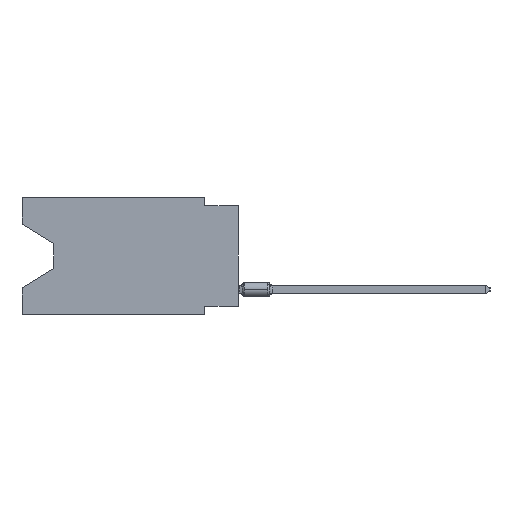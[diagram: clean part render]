
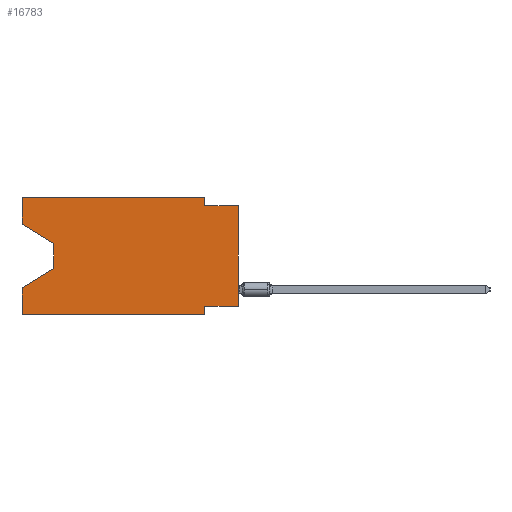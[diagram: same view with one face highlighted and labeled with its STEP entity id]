
A CAD part, left-side view. The second image highlights one B-rep face of the part: STEP entity #16783.
In plain terms, the highlighted planar face has unit normal (-1, 0, 0).
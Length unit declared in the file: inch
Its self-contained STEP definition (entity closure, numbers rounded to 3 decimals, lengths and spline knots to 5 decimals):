
#1095 = CARTESIAN_POINT ( 'NONE',  ( 0., 0.645, -0.08025 ) ) ;
#1118 = DIRECTION ( 'NONE',  ( 1., 0., 0. ) ) ;
#2425 = LINE ( 'NONE', #16137, #8555 ) ;
#2552 = ORIENTED_EDGE ( 'NONE', *, *, #15992, .T. ) ;
#2646 = ORIENTED_EDGE ( 'NONE', *, *, #29929, .T. ) ;
#3813 = VERTEX_POINT ( 'NONE', #6729 ) ;
#3839 = EDGE_CURVE ( 'NONE', #11808, #28434, #25571, .T. ) ;
#3952 = ORIENTED_EDGE ( 'NONE', *, *, #35474, .F. ) ;
#4165 = LINE ( 'NONE', #7543, #12275 ) ;
#4410 = VECTOR ( 'NONE', #7138, 39.37008 ) ;
#4477 = VERTEX_POINT ( 'NONE', #25203 ) ;
#5795 = VERTEX_POINT ( 'NONE', #40261 ) ;
#6729 = CARTESIAN_POINT ( 'NONE',  ( 0., 0.645, -0.35 ) ) ;
#7031 = CARTESIAN_POINT ( 'NONE',  ( 0., 0.1, -0.325 ) ) ;
#7138 = DIRECTION ( 'NONE',  ( 0., 0.855, -0.519 ) ) ;
#7151 = VECTOR ( 'NONE', #32783, 39.37008 ) ;
#7543 = CARTESIAN_POINT ( 'NONE',  ( 0., 0., -0.325 ) ) ;
#7919 = VECTOR ( 'NONE', #15474, 39.37008 ) ;
#8436 = VERTEX_POINT ( 'NONE', #17991 ) ;
#8555 = VECTOR ( 'NONE', #9391, 39.37008 ) ;
#8672 = DIRECTION ( 'NONE',  ( 0., 0., -1. ) ) ;
#9215 = LINE ( 'NONE', #25843, #41463 ) ;
#9391 = DIRECTION ( 'NONE',  ( 0., -1., 0. ) ) ;
#9828 = CARTESIAN_POINT ( 'NONE',  ( 0., 0.645, -0.35 ) ) ;
#10134 = VECTOR ( 'NONE', #16498, 39.37008 ) ;
#10283 = EDGE_CURVE ( 'NONE', #28434, #26085, #20039, .T. ) ;
#11442 = DIRECTION ( 'NONE',  ( 0., 0., -1. ) ) ;
#11808 = VERTEX_POINT ( 'NONE', #31929 ) ;
#11951 = LINE ( 'NONE', #22292, #36315 ) ;
#12116 = EDGE_CURVE ( 'NONE', #3813, #20471, #11951, .T. ) ;
#12165 = VERTEX_POINT ( 'NONE', #12174 ) ;
#12174 = CARTESIAN_POINT ( 'NONE',  ( 0., 0., -0.025 ) ) ;
#12275 = VECTOR ( 'NONE', #17874, 39.37008 ) ;
#12351 = LINE ( 'NONE', #16397, #17663 ) ;
#14331 = CARTESIAN_POINT ( 'NONE',  ( 0., 0.55, -0.212 ) ) ;
#14391 = EDGE_LOOP ( 'NONE', ( #43302, #19746, #2552, #34484, #2646, #43691, #32975, #43054, #3952, #27540, #29737, #34236 ) ) ;
#15425 = CARTESIAN_POINT ( 'NONE',  ( 0., 0.1, 0. ) ) ;
#15474 = DIRECTION ( 'NONE',  ( 0., -0.855, -0.519 ) ) ;
#15992 = EDGE_CURVE ( 'NONE', #26085, #20471, #37938, .T. ) ;
#16137 = CARTESIAN_POINT ( 'NONE',  ( 0., 0.645, 0. ) ) ;
#16397 = CARTESIAN_POINT ( 'NONE',  ( 0., 0., -0.025 ) ) ;
#16498 = DIRECTION ( 'NONE',  ( 0., 0., -1. ) ) ;
#16783 = ADVANCED_FACE ( 'NONE', ( #21348 ), #28104, .F. ) ;
#16889 = EDGE_CURVE ( 'NONE', #11808, #43099, #33010, .T. ) ;
#17663 = VECTOR ( 'NONE', #26286, 39.37008 ) ;
#17874 = DIRECTION ( 'NONE',  ( 0., 1., 0. ) ) ;
#17991 = CARTESIAN_POINT ( 'NONE',  ( 0., 0.1, -0.025 ) ) ;
#18970 = CARTESIAN_POINT ( 'NONE',  ( 0., 0.645, -0.26975 ) ) ;
#19081 = CARTESIAN_POINT ( 'NONE',  ( 0., 0.645, 0. ) ) ;
#19099 = DIRECTION ( 'NONE',  ( 0., 0., 1. ) ) ;
#19746 = ORIENTED_EDGE ( 'NONE', *, *, #10283, .T. ) ;
#20039 = LINE ( 'NONE', #20257, #42681 ) ;
#20257 = CARTESIAN_POINT ( 'NONE',  ( 0., 0.55, -0.138 ) ) ;
#20348 = EDGE_CURVE ( 'NONE', #4477, #39757, #4165, .T. ) ;
#20417 = EDGE_CURVE ( 'NONE', #39757, #23205, #22569, .T. ) ;
#20471 = VERTEX_POINT ( 'NONE', #18970 ) ;
#20620 = CARTESIAN_POINT ( 'NONE',  ( 0., 0.645, 0. ) ) ;
#20671 = VECTOR ( 'NONE', #8672, 39.37008 ) ;
#20800 = AXIS2_PLACEMENT_3D ( 'NONE', #31906, #1118, #11442 ) ;
#21058 = LINE ( 'NONE', #9828, #32996 ) ;
#21348 = FACE_OUTER_BOUND ( 'NONE', #14391, .T. ) ;
#21629 = DIRECTION ( 'NONE',  ( 0., 0., 1. ) ) ;
#22292 = CARTESIAN_POINT ( 'NONE',  ( 0., 0.645, 0. ) ) ;
#22569 = LINE ( 'NONE', #25938, #10134 ) ;
#23205 = VERTEX_POINT ( 'NONE', #41744 ) ;
#23768 = DIRECTION ( 'NONE',  ( 0., -1., 0. ) ) ;
#25203 = CARTESIAN_POINT ( 'NONE',  ( 0., 0., -0.325 ) ) ;
#25571 = LINE ( 'NONE', #1095, #7919 ) ;
#25843 = CARTESIAN_POINT ( 'NONE',  ( 0., 0., 0. ) ) ;
#25938 = CARTESIAN_POINT ( 'NONE',  ( 0., 0.1, -0.35 ) ) ;
#26085 = VERTEX_POINT ( 'NONE', #39390 ) ;
#26286 = DIRECTION ( 'NONE',  ( 0., -1., 0. ) ) ;
#26976 = CARTESIAN_POINT ( 'NONE',  ( 0., 0.55, -0.138 ) ) ;
#27540 = ORIENTED_EDGE ( 'NONE', *, *, #38713, .F. ) ;
#28104 = PLANE ( 'NONE',  #20800 ) ;
#28434 = VERTEX_POINT ( 'NONE', #26976 ) ;
#29579 = LINE ( 'NONE', #15425, #20671 ) ;
#29662 = EDGE_CURVE ( 'NONE', #43099, #5795, #2425, .T. ) ;
#29737 = ORIENTED_EDGE ( 'NONE', *, *, #29662, .F. ) ;
#29929 = EDGE_CURVE ( 'NONE', #3813, #23205, #21058, .T. ) ;
#31906 = CARTESIAN_POINT ( 'NONE',  ( 0., 0.645, 0. ) ) ;
#31929 = CARTESIAN_POINT ( 'NONE',  ( 0., 0.645, -0.08025 ) ) ;
#32783 = DIRECTION ( 'NONE',  ( 0., 0., 1. ) ) ;
#32975 = ORIENTED_EDGE ( 'NONE', *, *, #20348, .F. ) ;
#32996 = VECTOR ( 'NONE', #23768, 39.37008 ) ;
#33010 = LINE ( 'NONE', #19081, #7151 ) ;
#34236 = ORIENTED_EDGE ( 'NONE', *, *, #16889, .F. ) ;
#34484 = ORIENTED_EDGE ( 'NONE', *, *, #12116, .F. ) ;
#35474 = EDGE_CURVE ( 'NONE', #8436, #12165, #12351, .T. ) ;
#36315 = VECTOR ( 'NONE', #21629, 39.37008 ) ;
#36648 = EDGE_CURVE ( 'NONE', #4477, #12165, #9215, .T. ) ;
#36668 = DIRECTION ( 'NONE',  ( 0., 0., -1. ) ) ;
#37938 = LINE ( 'NONE', #14331, #4410 ) ;
#38713 = EDGE_CURVE ( 'NONE', #5795, #8436, #29579, .T. ) ;
#39390 = CARTESIAN_POINT ( 'NONE',  ( 0., 0.55, -0.212 ) ) ;
#39757 = VERTEX_POINT ( 'NONE', #7031 ) ;
#40261 = CARTESIAN_POINT ( 'NONE',  ( 0., 0.1, 0. ) ) ;
#41463 = VECTOR ( 'NONE', #19099, 39.37008 ) ;
#41744 = CARTESIAN_POINT ( 'NONE',  ( 0., 0.1, -0.35 ) ) ;
#42681 = VECTOR ( 'NONE', #36668, 39.37008 ) ;
#43054 = ORIENTED_EDGE ( 'NONE', *, *, #36648, .T. ) ;
#43099 = VERTEX_POINT ( 'NONE', #20620 ) ;
#43302 = ORIENTED_EDGE ( 'NONE', *, *, #3839, .T. ) ;
#43691 = ORIENTED_EDGE ( 'NONE', *, *, #20417, .F. ) ;
